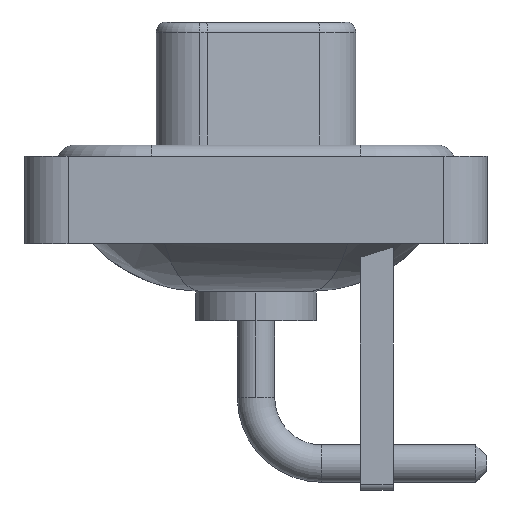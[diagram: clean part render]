
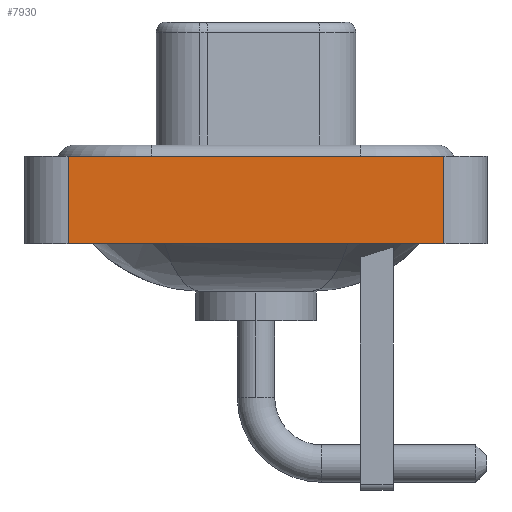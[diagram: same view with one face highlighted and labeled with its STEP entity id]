
A CAD part, left-side view. The second image highlights one B-rep face of the part: STEP entity #7930.
In plain terms, the highlighted planar face has unit normal (-1, 0, 0).
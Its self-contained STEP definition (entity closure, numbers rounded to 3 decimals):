
#18 = VECTOR ( 'NONE', #2204, 1000. ) ;
#601 = VERTEX_POINT ( 'NONE', #11691 ) ;
#676 = EDGE_LOOP ( 'NONE', ( #14547, #17299, #12845, #9638 ) ) ;
#2204 = DIRECTION ( 'NONE',  ( 0., 0., 1. ) ) ;
#3322 = EDGE_CURVE ( 'NONE', #601, #10957, #3948, .T. ) ;
#3948 = LINE ( 'NONE', #15383, #8916 ) ;
#4859 = DIRECTION ( 'NONE',  ( 0., 0., 1. ) ) ;
#5133 = VECTOR ( 'NONE', #10655, 1000. ) ;
#5810 = FACE_OUTER_BOUND ( 'NONE', #676, .T. ) ;
#6823 = VERTEX_POINT ( 'NONE', #16891 ) ;
#7369 = LINE ( 'NONE', #13070, #5133 ) ;
#7861 = LINE ( 'NONE', #10717, #10843 ) ;
#7930 = ADVANCED_FACE ( 'NONE', ( #5810 ), #9029, .T. ) ;
#8916 = VECTOR ( 'NONE', #13891, 1000. ) ;
#9029 = PLANE ( 'NONE',  #17944 ) ;
#9638 = ORIENTED_EDGE ( 'NONE', *, *, #12453, .T. ) ;
#10012 = VERTEX_POINT ( 'NONE', #16955 ) ;
#10170 = CARTESIAN_POINT ( 'NONE',  ( -7.25, -8.55, -3.6 ) ) ;
#10655 = DIRECTION ( 'NONE',  ( 0., -1., 0. ) ) ;
#10717 = CARTESIAN_POINT ( 'NONE',  ( -7.25, 8.55, -3.6 ) ) ;
#10843 = VECTOR ( 'NONE', #4859, 1000. ) ;
#10957 = VERTEX_POINT ( 'NONE', #15759 ) ;
#11691 = CARTESIAN_POINT ( 'NONE',  ( -7.25, 8.55, 0.4 ) ) ;
#11948 = CARTESIAN_POINT ( 'NONE',  ( -7.25, -8.55, -3.6 ) ) ;
#12098 = EDGE_CURVE ( 'NONE', #10012, #10957, #16558, .T. ) ;
#12453 = EDGE_CURVE ( 'NONE', #6823, #10012, #7369, .T. ) ;
#12845 = ORIENTED_EDGE ( 'NONE', *, *, #14840, .F. ) ;
#13070 = CARTESIAN_POINT ( 'NONE',  ( -7.25, -8.55, -3.6 ) ) ;
#13891 = DIRECTION ( 'NONE',  ( 0., -1., 0. ) ) ;
#14547 = ORIENTED_EDGE ( 'NONE', *, *, #12098, .T. ) ;
#14840 = EDGE_CURVE ( 'NONE', #6823, #601, #7861, .T. ) ;
#15383 = CARTESIAN_POINT ( 'NONE',  ( -7.25, -8.55, 0.4 ) ) ;
#15759 = CARTESIAN_POINT ( 'NONE',  ( -7.25, -8.55, 0.4 ) ) ;
#15938 = DIRECTION ( 'NONE',  ( -1., 0., 0. ) ) ;
#16110 = DIRECTION ( 'NONE',  ( 0., 0., 1. ) ) ;
#16558 = LINE ( 'NONE', #11948, #18 ) ;
#16891 = CARTESIAN_POINT ( 'NONE',  ( -7.25, 8.55, -3.6 ) ) ;
#16955 = CARTESIAN_POINT ( 'NONE',  ( -7.25, -8.55, -3.6 ) ) ;
#17299 = ORIENTED_EDGE ( 'NONE', *, *, #3322, .F. ) ;
#17944 = AXIS2_PLACEMENT_3D ( 'NONE', #10170, #15938, #16110 ) ;
